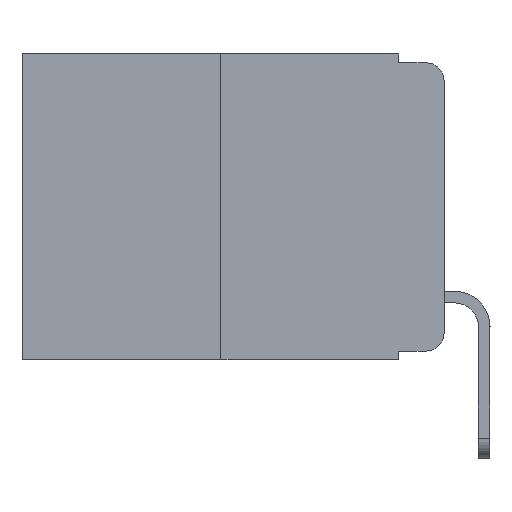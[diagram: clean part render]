
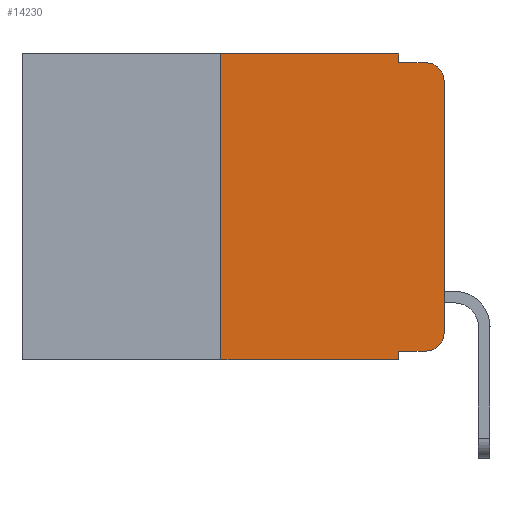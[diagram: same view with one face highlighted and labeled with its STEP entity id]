
A CAD part, left-side view. The second image highlights one B-rep face of the part: STEP entity #14230.
In plain terms, the highlighted planar face has unit normal (-1, 0, 0).
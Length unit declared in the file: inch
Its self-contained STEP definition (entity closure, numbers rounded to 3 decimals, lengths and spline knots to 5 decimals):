
#442 = LINE ( 'NONE', #11204, #15553 ) ;
#525 = DIRECTION ( 'NONE',  ( 0., -1., 0. ) ) ;
#606 = ORIENTED_EDGE ( 'NONE', *, *, #7449, .T. ) ;
#925 = CARTESIAN_POINT ( 'NONE',  ( 0., 0.051, -0.333 ) ) ;
#998 = EDGE_CURVE ( 'NONE', #9331, #11114, #17924, .T. ) ;
#1346 = CARTESIAN_POINT ( 'NONE',  ( 0., 0.25, 0. ) ) ;
#1780 = CARTESIAN_POINT ( 'NONE',  ( 0., 0.051, 0. ) ) ;
#2363 = EDGE_CURVE ( 'NONE', #13573, #19407, #22230, .T. ) ;
#3091 = LINE ( 'NONE', #22297, #5719 ) ;
#3494 = VECTOR ( 'NONE', #525, 39.37008 ) ;
#3665 = DIRECTION ( 'NONE',  ( -1., 0., 0. ) ) ;
#3782 = CARTESIAN_POINT ( 'NONE',  ( 0., 0., 0. ) ) ;
#3856 = AXIS2_PLACEMENT_3D ( 'NONE', #19364, #3665, #10651 ) ;
#4081 = DIRECTION ( 'NONE',  ( 0., -1., 0. ) ) ;
#4467 = DIRECTION ( 'NONE',  ( 0., 0., 1. ) ) ;
#4625 = DIRECTION ( 'NONE',  ( 0., -1., 0. ) ) ;
#4739 = VECTOR ( 'NONE', #13747, 39.37008 ) ;
#4788 = VERTEX_POINT ( 'NONE', #21879 ) ;
#5152 = ORIENTED_EDGE ( 'NONE', *, *, #17704, .T. ) ;
#5719 = VECTOR ( 'NONE', #4467, 39.37008 ) ;
#5919 = CARTESIAN_POINT ( 'NONE',  ( 0., 0.02, -0.03 ) ) ;
#6857 = VECTOR ( 'NONE', #4625, 39.37008 ) ;
#6898 = ORIENTED_EDGE ( 'NONE', *, *, #19226, .F. ) ;
#7449 = EDGE_CURVE ( 'NONE', #18161, #12140, #22108, .T. ) ;
#7500 = CARTESIAN_POINT ( 'NONE',  ( 0., 0.473, 0. ) ) ;
#7815 = PLANE ( 'NONE',  #15020 ) ;
#7914 = ORIENTED_EDGE ( 'NONE', *, *, #19108, .F. ) ;
#8313 = LINE ( 'NONE', #11645, #15569 ) ;
#8771 = VERTEX_POINT ( 'NONE', #925 ) ;
#9241 = EDGE_CURVE ( 'NONE', #4788, #19959, #11946, .T. ) ;
#9331 = VERTEX_POINT ( 'NONE', #1346 ) ;
#9459 = VECTOR ( 'NONE', #21278, 39.37008 ) ;
#9926 = DIRECTION ( 'NONE',  ( 0., -1., 0. ) ) ;
#9933 = ORIENTED_EDGE ( 'NONE', *, *, #2363, .T. ) ;
#10500 = CARTESIAN_POINT ( 'NONE',  ( 0., 0.051, -0.333 ) ) ;
#10651 = DIRECTION ( 'NONE',  ( 0., 0., -1. ) ) ;
#10685 = CARTESIAN_POINT ( 'NONE',  ( 0., 0.02, -0.333 ) ) ;
#10865 = DIRECTION ( 'NONE',  ( 0., 0., -1. ) ) ;
#11114 = VERTEX_POINT ( 'NONE', #1780 ) ;
#11147 = DIRECTION ( 'NONE',  ( 0., 0., -1. ) ) ;
#11204 = CARTESIAN_POINT ( 'NONE',  ( 0., 0.051, 0. ) ) ;
#11217 = ORIENTED_EDGE ( 'NONE', *, *, #998, .F. ) ;
#11384 = CARTESIAN_POINT ( 'NONE',  ( 0., 0.473, -0.343 ) ) ;
#11645 = CARTESIAN_POINT ( 'NONE',  ( 0., 0.051, -0.01 ) ) ;
#11946 = CIRCLE ( 'NONE', #21801, 0.02 ) ;
#12140 = VERTEX_POINT ( 'NONE', #20239 ) ;
#12472 = LINE ( 'NONE', #3782, #9459 ) ;
#12985 = EDGE_LOOP ( 'NONE', ( #15105, #15951, #6898, #19429, #11217, #13315, #9933, #7914, #5152, #606 ) ) ;
#13130 = DIRECTION ( 'NONE',  ( -1., 0., 0. ) ) ;
#13257 = EDGE_CURVE ( 'NONE', #11114, #18206, #15478, .T. ) ;
#13306 = FACE_OUTER_BOUND ( 'NONE', #12985, .T. ) ;
#13315 = ORIENTED_EDGE ( 'NONE', *, *, #18930, .F. ) ;
#13573 = VERTEX_POINT ( 'NONE', #20818 ) ;
#13747 = DIRECTION ( 'NONE',  ( 0., 0., -1. ) ) ;
#14230 = ADVANCED_FACE ( 'NONE', ( #13306 ), #7815, .F. ) ;
#14317 = CARTESIAN_POINT ( 'NONE',  ( 0., 0.051, -0.01 ) ) ;
#14920 = CARTESIAN_POINT ( 'NONE',  ( 0., 0.473, 0. ) ) ;
#15020 = AXIS2_PLACEMENT_3D ( 'NONE', #14920, #21887, #11147 ) ;
#15105 = ORIENTED_EDGE ( 'NONE', *, *, #22608, .T. ) ;
#15428 = CARTESIAN_POINT ( 'NONE',  ( 0., 0.051, -0.343 ) ) ;
#15478 = LINE ( 'NONE', #18803, #4739 ) ;
#15553 = VECTOR ( 'NONE', #10865, 39.37008 ) ;
#15569 = VECTOR ( 'NONE', #9926, 39.37008 ) ;
#15758 = LINE ( 'NONE', #10500, #3494 ) ;
#15951 = ORIENTED_EDGE ( 'NONE', *, *, #9241, .T. ) ;
#16344 = DIRECTION ( 'NONE',  ( 0., 0., -1. ) ) ;
#17491 = CARTESIAN_POINT ( 'NONE',  ( 0., 0.02, -0.01 ) ) ;
#17704 = EDGE_CURVE ( 'NONE', #8771, #18161, #15758, .T. ) ;
#17924 = LINE ( 'NONE', #7500, #22141 ) ;
#18161 = VERTEX_POINT ( 'NONE', #10685 ) ;
#18206 = VERTEX_POINT ( 'NONE', #14317 ) ;
#18803 = CARTESIAN_POINT ( 'NONE',  ( 0., 0.051, 0. ) ) ;
#18930 = EDGE_CURVE ( 'NONE', #13573, #9331, #3091, .T. ) ;
#19108 = EDGE_CURVE ( 'NONE', #8771, #19407, #442, .T. ) ;
#19226 = EDGE_CURVE ( 'NONE', #18206, #19959, #8313, .T. ) ;
#19364 = CARTESIAN_POINT ( 'NONE',  ( 0., 0.02, -0.313 ) ) ;
#19407 = VERTEX_POINT ( 'NONE', #15428 ) ;
#19429 = ORIENTED_EDGE ( 'NONE', *, *, #13257, .F. ) ;
#19959 = VERTEX_POINT ( 'NONE', #17491 ) ;
#20239 = CARTESIAN_POINT ( 'NONE',  ( 0., 0., -0.313 ) ) ;
#20818 = CARTESIAN_POINT ( 'NONE',  ( 0., 0.25, -0.343 ) ) ;
#21278 = DIRECTION ( 'NONE',  ( 0., 0., 1. ) ) ;
#21801 = AXIS2_PLACEMENT_3D ( 'NONE', #5919, #13130, #16344 ) ;
#21879 = CARTESIAN_POINT ( 'NONE',  ( 0., 0., -0.03 ) ) ;
#21887 = DIRECTION ( 'NONE',  ( 1., 0., 0. ) ) ;
#22108 = CIRCLE ( 'NONE', #3856, 0.02 ) ;
#22141 = VECTOR ( 'NONE', #4081, 39.37008 ) ;
#22230 = LINE ( 'NONE', #11384, #6857 ) ;
#22297 = CARTESIAN_POINT ( 'NONE',  ( 0., 0.25, 0. ) ) ;
#22608 = EDGE_CURVE ( 'NONE', #12140, #4788, #12472, .T. ) ;
